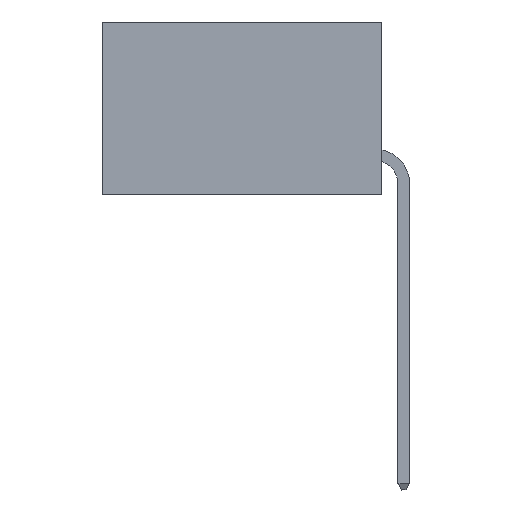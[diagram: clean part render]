
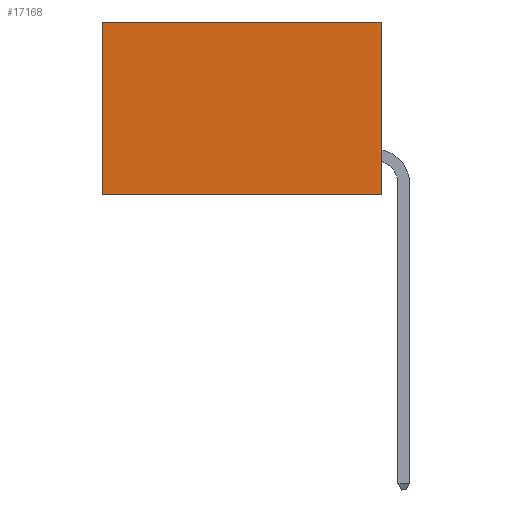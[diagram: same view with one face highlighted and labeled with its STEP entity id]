
A CAD part, left-side view. The second image highlights one B-rep face of the part: STEP entity #17168.
In plain terms, the highlighted planar face has unit normal (-1, 0, 0).
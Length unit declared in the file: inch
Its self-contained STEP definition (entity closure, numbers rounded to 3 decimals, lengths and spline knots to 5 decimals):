
#874 = DIRECTION ( 'NONE',  ( 0., 1., 0. ) ) ;
#908 = VECTOR ( 'NONE', #8279, 39.37008 ) ;
#994 = EDGE_CURVE ( 'NONE', #9907, #14785, #13276, .T. ) ;
#1121 = PLANE ( 'NONE',  #15513 ) ;
#1253 = VECTOR ( 'NONE', #8295, 39.37008 ) ;
#2170 = ORIENTED_EDGE ( 'NONE', *, *, #9283, .F. ) ;
#2309 = EDGE_CURVE ( 'NONE', #14785, #8043, #17321, .T. ) ;
#2392 = CARTESIAN_POINT ( 'NONE',  ( 0.2875, 0.6, -0.37 ) ) ;
#2648 = CARTESIAN_POINT ( 'NONE',  ( 0.2875, 0.6, 0. ) ) ;
#3220 = LINE ( 'NONE', #15488, #908 ) ;
#4188 = CARTESIAN_POINT ( 'NONE',  ( 0.2875, 0., -0.37 ) ) ;
#4644 = EDGE_CURVE ( 'NONE', #15494, #8043, #3220, .T. ) ;
#5496 = CARTESIAN_POINT ( 'NONE',  ( 0.2875, 0., 0. ) ) ;
#5765 = ORIENTED_EDGE ( 'NONE', *, *, #4644, .F. ) ;
#6097 = ORIENTED_EDGE ( 'NONE', *, *, #994, .T. ) ;
#6763 = DIRECTION ( 'NONE',  ( 1., 0., 0. ) ) ;
#7271 = DIRECTION ( 'NONE',  ( 0., 0., -1. ) ) ;
#8043 = VERTEX_POINT ( 'NONE', #2392 ) ;
#8279 = DIRECTION ( 'NONE',  ( 0., 1., 0. ) ) ;
#8295 = DIRECTION ( 'NONE',  ( 0., 0., -1. ) ) ;
#8566 = VECTOR ( 'NONE', #7271, 39.37008 ) ;
#8690 = ORIENTED_EDGE ( 'NONE', *, *, #2309, .T. ) ;
#9283 = EDGE_CURVE ( 'NONE', #9907, #15494, #9972, .T. ) ;
#9887 = CARTESIAN_POINT ( 'NONE',  ( 0.2875, 0., 0. ) ) ;
#9907 = VERTEX_POINT ( 'NONE', #9887 ) ;
#9972 = LINE ( 'NONE', #11211, #1253 ) ;
#10977 = CARTESIAN_POINT ( 'NONE',  ( 0.2875, 0., 0. ) ) ;
#11211 = CARTESIAN_POINT ( 'NONE',  ( 0.2875, 0., 0. ) ) ;
#11582 = FACE_OUTER_BOUND ( 'NONE', #15078, .T. ) ;
#11633 = VECTOR ( 'NONE', #874, 39.37008 ) ;
#13276 = LINE ( 'NONE', #10977, #11633 ) ;
#14785 = VERTEX_POINT ( 'NONE', #16581 ) ;
#15078 = EDGE_LOOP ( 'NONE', ( #8690, #5765, #2170, #6097 ) ) ;
#15488 = CARTESIAN_POINT ( 'NONE',  ( 0.2875, 0., -0.37 ) ) ;
#15494 = VERTEX_POINT ( 'NONE', #4188 ) ;
#15513 = AXIS2_PLACEMENT_3D ( 'NONE', #5496, #6763, #15763 ) ;
#15763 = DIRECTION ( 'NONE',  ( 0., 0., -1. ) ) ;
#16581 = CARTESIAN_POINT ( 'NONE',  ( 0.2875, 0.6, 0. ) ) ;
#17168 = ADVANCED_FACE ( 'NONE', ( #11582 ), #1121, .F. ) ;
#17321 = LINE ( 'NONE', #2648, #8566 ) ;
